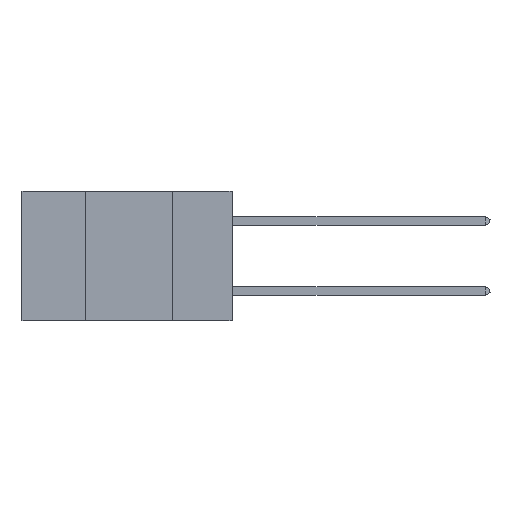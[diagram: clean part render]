
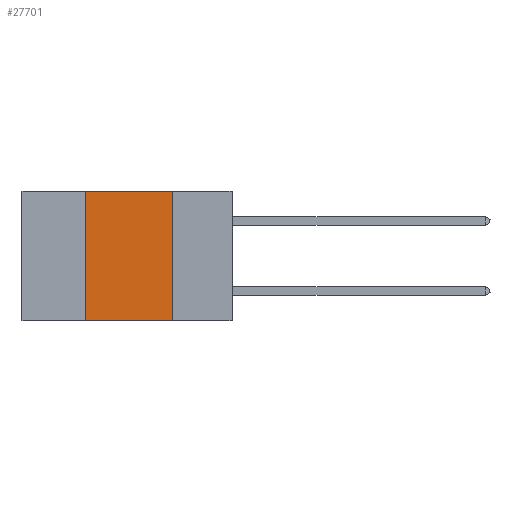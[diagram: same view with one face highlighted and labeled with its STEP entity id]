
A CAD part, left-side view. The second image highlights one B-rep face of the part: STEP entity #27701.
In plain terms, the highlighted planar face has unit normal (-1, 0, 0).
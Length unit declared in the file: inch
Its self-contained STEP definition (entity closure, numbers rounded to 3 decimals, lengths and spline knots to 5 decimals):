
#103 = DIRECTION ( 'NONE',  ( 1., 0., 0. ) ) ;
#2954 = CARTESIAN_POINT ( 'NONE',  ( 0., 0.17, 0. ) ) ;
#2995 = DIRECTION ( 'NONE',  ( 0., -1., 0. ) ) ;
#4210 = VECTOR ( 'NONE', #20550, 39.37008 ) ;
#4737 = AXIS2_PLACEMENT_3D ( 'NONE', #15923, #103, #18521 ) ;
#5277 = VECTOR ( 'NONE', #2995, 39.37008 ) ;
#6681 = EDGE_CURVE ( 'NONE', #19797, #19765, #31194, .T. ) ;
#7397 = ORIENTED_EDGE ( 'NONE', *, *, #6681, .T. ) ;
#7493 = ORIENTED_EDGE ( 'NONE', *, *, #24025, .F. ) ;
#7520 = ORIENTED_EDGE ( 'NONE', *, *, #12607, .F. ) ;
#7533 = VERTEX_POINT ( 'NONE', #19287 ) ;
#7771 = LINE ( 'NONE', #21984, #27599 ) ;
#7857 = ORIENTED_EDGE ( 'NONE', *, *, #10865, .F. ) ;
#8648 = VERTEX_POINT ( 'NONE', #20103 ) ;
#8966 = CARTESIAN_POINT ( 'NONE',  ( 0., 0.42, -0.37 ) ) ;
#10817 = DIRECTION ( 'NONE',  ( 0., 0., -1. ) ) ;
#10865 = EDGE_CURVE ( 'NONE', #7533, #19765, #13189, .T. ) ;
#12607 = EDGE_CURVE ( 'NONE', #19797, #8648, #18935, .T. ) ;
#13189 = LINE ( 'NONE', #2954, #32883 ) ;
#13289 = PLANE ( 'NONE',  #4737 ) ;
#14102 = CARTESIAN_POINT ( 'NONE',  ( 0., 0.17, -0.37 ) ) ;
#15923 = CARTESIAN_POINT ( 'NONE',  ( 0., 0.6, 0. ) ) ;
#17307 = EDGE_LOOP ( 'NONE', ( #7857, #7493, #7520, #7397 ) ) ;
#18021 = CARTESIAN_POINT ( 'NONE',  ( 0., 0.42, 0. ) ) ;
#18521 = DIRECTION ( 'NONE',  ( 0., 0., -1. ) ) ;
#18935 = LINE ( 'NONE', #18021, #4210 ) ;
#19287 = CARTESIAN_POINT ( 'NONE',  ( 0., 0.17, 0. ) ) ;
#19765 = VERTEX_POINT ( 'NONE', #14102 ) ;
#19797 = VERTEX_POINT ( 'NONE', #8966 ) ;
#20103 = CARTESIAN_POINT ( 'NONE',  ( 0., 0.42, 0. ) ) ;
#20550 = DIRECTION ( 'NONE',  ( 0., 0., 1. ) ) ;
#21984 = CARTESIAN_POINT ( 'NONE',  ( 0., 0.6, 0. ) ) ;
#22972 = FACE_OUTER_BOUND ( 'NONE', #17307, .T. ) ;
#24025 = EDGE_CURVE ( 'NONE', #8648, #7533, #7771, .T. ) ;
#27149 = DIRECTION ( 'NONE',  ( 0., -1., 0. ) ) ;
#27599 = VECTOR ( 'NONE', #27149, 39.37008 ) ;
#27701 = ADVANCED_FACE ( 'NONE', ( #22972 ), #13289, .F. ) ;
#31194 = LINE ( 'NONE', #31458, #5277 ) ;
#31458 = CARTESIAN_POINT ( 'NONE',  ( 0., 0.6, -0.37 ) ) ;
#32883 = VECTOR ( 'NONE', #10817, 39.37008 ) ;
